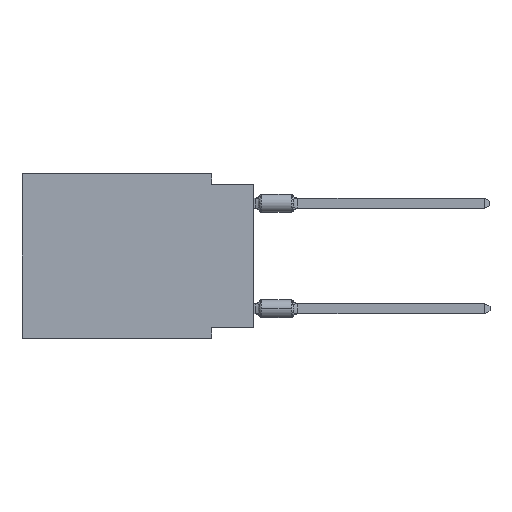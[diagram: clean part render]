
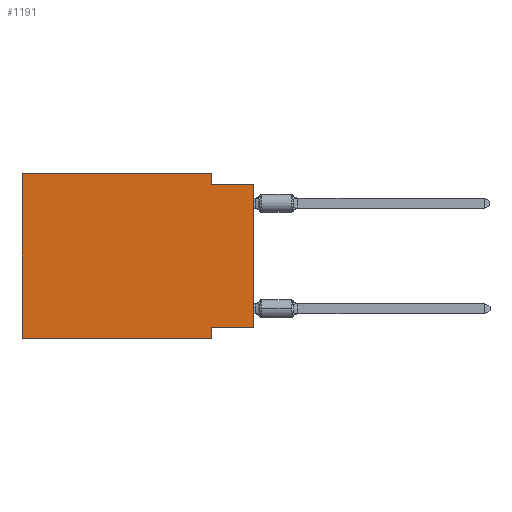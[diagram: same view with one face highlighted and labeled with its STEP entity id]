
A CAD part, left-side view. The second image highlights one B-rep face of the part: STEP entity #1191.
In plain terms, the highlighted planar face has unit normal (-1, 0, 0).
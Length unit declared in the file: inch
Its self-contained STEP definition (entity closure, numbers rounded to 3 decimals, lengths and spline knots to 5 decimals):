
#990 = VECTOR ( 'NONE', #31210, 39.37008 ) ;
#1191 = ADVANCED_FACE ( 'NONE', ( #5975 ), #13730, .F. ) ;
#1701 = CARTESIAN_POINT ( 'NONE',  ( 0., 0.55, 0. ) ) ;
#2084 = VECTOR ( 'NONE', #53796, 39.37008 ) ;
#2202 = CARTESIAN_POINT ( 'NONE',  ( 0., 0.1, -0.39 ) ) ;
#3483 = CARTESIAN_POINT ( 'NONE',  ( 0., 0.55, 0. ) ) ;
#4773 = VERTEX_POINT ( 'NONE', #5644 ) ;
#5644 = CARTESIAN_POINT ( 'NONE',  ( 0., 0.55, -0.39 ) ) ;
#5724 = DIRECTION ( 'NONE',  ( 1., 0., 0. ) ) ;
#5975 = FACE_OUTER_BOUND ( 'NONE', #33736, .T. ) ;
#6042 = VECTOR ( 'NONE', #48210, 39.37008 ) ;
#6124 = VECTOR ( 'NONE', #50100, 39.37008 ) ;
#6251 = DIRECTION ( 'NONE',  ( 0., 0., -1. ) ) ;
#6865 = CARTESIAN_POINT ( 'NONE',  ( 0., 0.1, -0.39 ) ) ;
#7325 = ORIENTED_EDGE ( 'NONE', *, *, #55364, .F. ) ;
#8069 = CARTESIAN_POINT ( 'NONE',  ( 0., 0.1, -0.365 ) ) ;
#10197 = VECTOR ( 'NONE', #27833, 39.37008 ) ;
#11442 = AXIS2_PLACEMENT_3D ( 'NONE', #1701, #5724, #6251 ) ;
#11495 = EDGE_CURVE ( 'NONE', #48280, #35248, #45965, .T. ) ;
#11725 = DIRECTION ( 'NONE',  ( 0., 0., -1. ) ) ;
#12483 = ORIENTED_EDGE ( 'NONE', *, *, #13203, .F. ) ;
#12999 = VERTEX_POINT ( 'NONE', #3483 ) ;
#13203 = EDGE_CURVE ( 'NONE', #12999, #28495, #36577, .T. ) ;
#13730 = PLANE ( 'NONE',  #11442 ) ;
#14050 = ORIENTED_EDGE ( 'NONE', *, *, #11495, .F. ) ;
#15105 = ORIENTED_EDGE ( 'NONE', *, *, #30870, .T. ) ;
#15281 = LINE ( 'NONE', #41519, #6124 ) ;
#18335 = CARTESIAN_POINT ( 'NONE',  ( 0., 0.1, 0. ) ) ;
#18983 = CARTESIAN_POINT ( 'NONE',  ( 0., 0., -0.365 ) ) ;
#20111 = LINE ( 'NONE', #33237, #39645 ) ;
#22090 = ORIENTED_EDGE ( 'NONE', *, *, #53079, .F. ) ;
#22111 = CARTESIAN_POINT ( 'NONE',  ( 0., 0., -0.025 ) ) ;
#22750 = ORIENTED_EDGE ( 'NONE', *, *, #55926, .F. ) ;
#23466 = CARTESIAN_POINT ( 'NONE',  ( 0., 0.55, 0. ) ) ;
#24444 = VECTOR ( 'NONE', #11725, 39.37008 ) ;
#24697 = DIRECTION ( 'NONE',  ( 0., 0., 1. ) ) ;
#27394 = LINE ( 'NONE', #30806, #6042 ) ;
#27833 = DIRECTION ( 'NONE',  ( 0., 0., 1. ) ) ;
#28495 = VERTEX_POINT ( 'NONE', #18335 ) ;
#30806 = CARTESIAN_POINT ( 'NONE',  ( 0., 0., -0.025 ) ) ;
#30870 = EDGE_CURVE ( 'NONE', #4773, #35248, #31482, .T. ) ;
#31210 = DIRECTION ( 'NONE',  ( 0., -1., 0. ) ) ;
#31482 = LINE ( 'NONE', #35765, #990 ) ;
#32027 = DIRECTION ( 'NONE',  ( 0., -1., 0. ) ) ;
#32303 = EDGE_CURVE ( 'NONE', #44246, #38529, #44665, .T. ) ;
#32377 = CARTESIAN_POINT ( 'NONE',  ( 0., 0., 0. ) ) ;
#33237 = CARTESIAN_POINT ( 'NONE',  ( 0., 0.55, 0. ) ) ;
#33314 = ORIENTED_EDGE ( 'NONE', *, *, #32303, .T. ) ;
#33501 = CARTESIAN_POINT ( 'NONE',  ( 0., 0., -0.365 ) ) ;
#33736 = EDGE_LOOP ( 'NONE', ( #33314, #7325, #22750, #12483, #22090, #15105, #14050, #47565 ) ) ;
#35248 = VERTEX_POINT ( 'NONE', #2202 ) ;
#35765 = CARTESIAN_POINT ( 'NONE',  ( 0., 0.55, -0.39 ) ) ;
#36577 = LINE ( 'NONE', #23466, #46122 ) ;
#38321 = EDGE_CURVE ( 'NONE', #44246, #48280, #40934, .T. ) ;
#38529 = VERTEX_POINT ( 'NONE', #22111 ) ;
#38684 = CARTESIAN_POINT ( 'NONE',  ( 0., 0.1, -0.025 ) ) ;
#39645 = VECTOR ( 'NONE', #24697, 39.37008 ) ;
#40934 = LINE ( 'NONE', #18983, #2084 ) ;
#41519 = CARTESIAN_POINT ( 'NONE',  ( 0., 0.1, 0. ) ) ;
#44246 = VERTEX_POINT ( 'NONE', #33501 ) ;
#44665 = LINE ( 'NONE', #32377, #10197 ) ;
#45965 = LINE ( 'NONE', #6865, #24444 ) ;
#46122 = VECTOR ( 'NONE', #32027, 39.37008 ) ;
#47565 = ORIENTED_EDGE ( 'NONE', *, *, #38321, .F. ) ;
#48210 = DIRECTION ( 'NONE',  ( 0., -1., 0. ) ) ;
#48280 = VERTEX_POINT ( 'NONE', #8069 ) ;
#50100 = DIRECTION ( 'NONE',  ( 0., 0., -1. ) ) ;
#52301 = VERTEX_POINT ( 'NONE', #38684 ) ;
#53079 = EDGE_CURVE ( 'NONE', #4773, #12999, #20111, .T. ) ;
#53796 = DIRECTION ( 'NONE',  ( 0., 1., 0. ) ) ;
#55364 = EDGE_CURVE ( 'NONE', #52301, #38529, #27394, .T. ) ;
#55926 = EDGE_CURVE ( 'NONE', #28495, #52301, #15281, .T. ) ;
